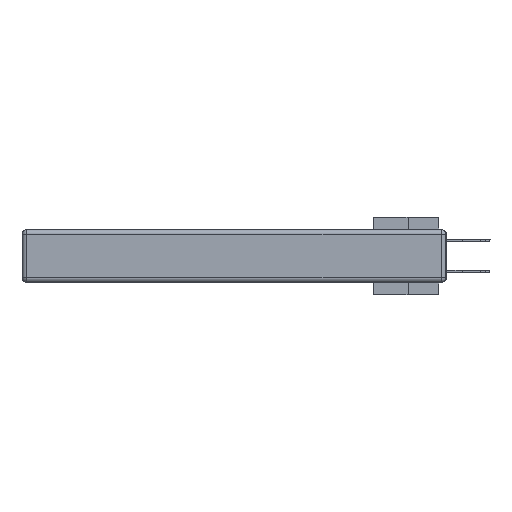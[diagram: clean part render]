
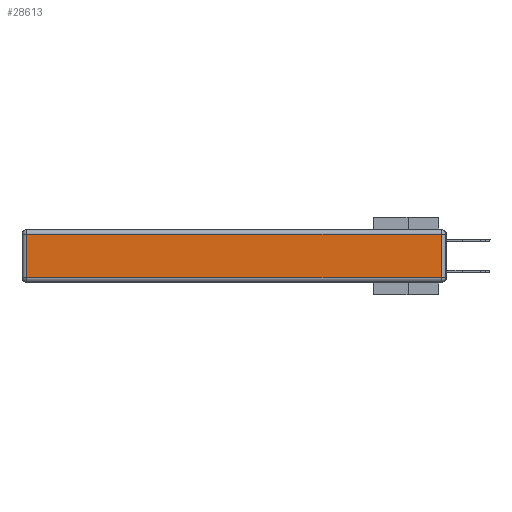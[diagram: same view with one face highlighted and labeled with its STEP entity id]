
A CAD part, left-side view. The second image highlights one B-rep face of the part: STEP entity #28613.
In plain terms, the highlighted planar face has unit normal (-1, 0, 0).
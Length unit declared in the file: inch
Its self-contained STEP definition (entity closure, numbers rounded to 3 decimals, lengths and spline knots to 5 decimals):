
#397 = EDGE_CURVE ( 'NONE', #31973, #20837, #21201, .T. ) ;
#439 = AXIS2_PLACEMENT_3D ( 'NONE', #2140, #19348, #19513 ) ;
#1412 = ORIENTED_EDGE ( 'NONE', *, *, #6074, .T. ) ;
#2140 = CARTESIAN_POINT ( 'NONE',  ( 0., 0., -0.343 ) ) ;
#2502 = LINE ( 'NONE', #17580, #11361 ) ;
#3147 = ORIENTED_EDGE ( 'NONE', *, *, #12926, .T. ) ;
#3277 = VERTEX_POINT ( 'NONE', #9863 ) ;
#3825 = CARTESIAN_POINT ( 'NONE',  ( 0., 0., -0.313 ) ) ;
#4157 = LINE ( 'NONE', #21888, #30057 ) ;
#6074 = EDGE_CURVE ( 'NONE', #13475, #3277, #13980, .T. ) ;
#6227 = DIRECTION ( 'NONE',  ( 0., 1., 0. ) ) ;
#8640 = CARTESIAN_POINT ( 'NONE',  ( 0., 2.72, -0.03 ) ) ;
#9863 = CARTESIAN_POINT ( 'NONE',  ( 0., 0.03, -0.313 ) ) ;
#10254 = VECTOR ( 'NONE', #28622, 39.37008 ) ;
#11361 = VECTOR ( 'NONE', #17256, 39.37008 ) ;
#12926 = EDGE_CURVE ( 'NONE', #3277, #31973, #4157, .T. ) ;
#13475 = VERTEX_POINT ( 'NONE', #27105 ) ;
#13980 = LINE ( 'NONE', #3825, #10254 ) ;
#17069 = CARTESIAN_POINT ( 'NONE',  ( 0., 0.03, -0.03 ) ) ;
#17256 = DIRECTION ( 'NONE',  ( 0., 0., -1. ) ) ;
#17580 = CARTESIAN_POINT ( 'NONE',  ( 0., 2.72, -0.343 ) ) ;
#18773 = VECTOR ( 'NONE', #6227, 39.37008 ) ;
#19089 = DIRECTION ( 'NONE',  ( 0., 0., 1. ) ) ;
#19348 = DIRECTION ( 'NONE',  ( -1., 0., 0. ) ) ;
#19513 = DIRECTION ( 'NONE',  ( 0., 0., 1. ) ) ;
#19909 = ORIENTED_EDGE ( 'NONE', *, *, #397, .T. ) ;
#20837 = VERTEX_POINT ( 'NONE', #8640 ) ;
#21201 = LINE ( 'NONE', #31232, #18773 ) ;
#21830 = PLANE ( 'NONE',  #439 ) ;
#21888 = CARTESIAN_POINT ( 'NONE',  ( 0., 0.03, -0.343 ) ) ;
#21905 = EDGE_CURVE ( 'NONE', #20837, #13475, #2502, .T. ) ;
#24297 = FACE_OUTER_BOUND ( 'NONE', #28554, .T. ) ;
#27105 = CARTESIAN_POINT ( 'NONE',  ( 0., 2.72, -0.313 ) ) ;
#28554 = EDGE_LOOP ( 'NONE', ( #1412, #3147, #19909, #29411 ) ) ;
#28613 = ADVANCED_FACE ( 'NONE', ( #24297 ), #21830, .T. ) ;
#28622 = DIRECTION ( 'NONE',  ( 0., -1., 0. ) ) ;
#29411 = ORIENTED_EDGE ( 'NONE', *, *, #21905, .T. ) ;
#30057 = VECTOR ( 'NONE', #19089, 39.37008 ) ;
#31232 = CARTESIAN_POINT ( 'NONE',  ( 0., 2.75, -0.03 ) ) ;
#31973 = VERTEX_POINT ( 'NONE', #17069 ) ;
